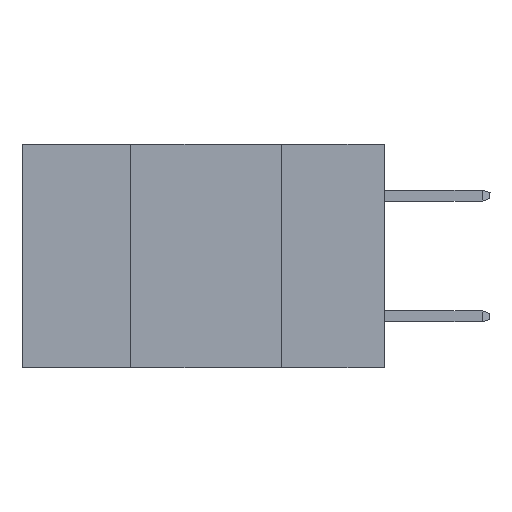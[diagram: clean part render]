
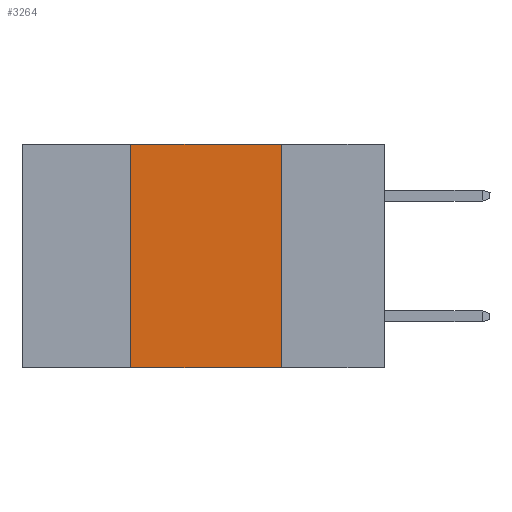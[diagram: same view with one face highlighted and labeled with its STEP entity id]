
A CAD part, left-side view. The second image highlights one B-rep face of the part: STEP entity #3264.
In plain terms, the highlighted planar face has unit normal (-1, 0, 0).
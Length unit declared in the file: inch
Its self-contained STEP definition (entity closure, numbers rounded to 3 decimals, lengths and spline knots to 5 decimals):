
#621 = DIRECTION ( 'NONE',  ( 0., -1., 0. ) ) ;
#633 = EDGE_CURVE ( 'NONE', #6293, #1462, #4921, .T. ) ;
#1462 = VERTEX_POINT ( 'NONE', #1983 ) ;
#1983 = CARTESIAN_POINT ( 'NONE',  ( 0., 0.17, -0.37 ) ) ;
#2547 = EDGE_CURVE ( 'NONE', #11130, #1462, #5592, .T. ) ;
#2587 = ORIENTED_EDGE ( 'NONE', *, *, #633, .F. ) ;
#2817 = ORIENTED_EDGE ( 'NONE', *, *, #6175, .F. ) ;
#3045 = VECTOR ( 'NONE', #10610, 39.37008 ) ;
#3264 = ADVANCED_FACE ( 'NONE', ( #13187 ), #14008, .F. ) ;
#4022 = VERTEX_POINT ( 'NONE', #5114 ) ;
#4921 = LINE ( 'NONE', #12921, #3045 ) ;
#5114 = CARTESIAN_POINT ( 'NONE',  ( 0., 0.42, 0. ) ) ;
#5224 = VECTOR ( 'NONE', #7426, 39.37008 ) ;
#5592 = LINE ( 'NONE', #10114, #11510 ) ;
#6175 = EDGE_CURVE ( 'NONE', #4022, #6293, #13709, .T. ) ;
#6293 = VERTEX_POINT ( 'NONE', #14101 ) ;
#6456 = VECTOR ( 'NONE', #621, 39.37008 ) ;
#6945 = CARTESIAN_POINT ( 'NONE',  ( 0., 0.42, -0.37 ) ) ;
#7426 = DIRECTION ( 'NONE',  ( 0., 0., 1. ) ) ;
#8776 = ORIENTED_EDGE ( 'NONE', *, *, #2547, .T. ) ;
#8911 = DIRECTION ( 'NONE',  ( 0., -1., 0. ) ) ;
#9613 = EDGE_LOOP ( 'NONE', ( #2587, #2817, #11838, #8776 ) ) ;
#10026 = CARTESIAN_POINT ( 'NONE',  ( 0., 0.6, 0. ) ) ;
#10114 = CARTESIAN_POINT ( 'NONE',  ( 0., 0.6, -0.37 ) ) ;
#10610 = DIRECTION ( 'NONE',  ( 0., 0., -1. ) ) ;
#10717 = EDGE_CURVE ( 'NONE', #11130, #4022, #11890, .T. ) ;
#11130 = VERTEX_POINT ( 'NONE', #6945 ) ;
#11450 = DIRECTION ( 'NONE',  ( 0., 0., -1. ) ) ;
#11503 = CARTESIAN_POINT ( 'NONE',  ( 0., 0.6, 0. ) ) ;
#11510 = VECTOR ( 'NONE', #8911, 39.37008 ) ;
#11665 = AXIS2_PLACEMENT_3D ( 'NONE', #11503, #12769, #11450 ) ;
#11838 = ORIENTED_EDGE ( 'NONE', *, *, #10717, .F. ) ;
#11890 = LINE ( 'NONE', #14590, #5224 ) ;
#12769 = DIRECTION ( 'NONE',  ( 1., 0., 0. ) ) ;
#12921 = CARTESIAN_POINT ( 'NONE',  ( 0., 0.17, 0. ) ) ;
#13187 = FACE_OUTER_BOUND ( 'NONE', #9613, .T. ) ;
#13709 = LINE ( 'NONE', #10026, #6456 ) ;
#14008 = PLANE ( 'NONE',  #11665 ) ;
#14101 = CARTESIAN_POINT ( 'NONE',  ( 0., 0.17, 0. ) ) ;
#14590 = CARTESIAN_POINT ( 'NONE',  ( 0., 0.42, 0. ) ) ;
